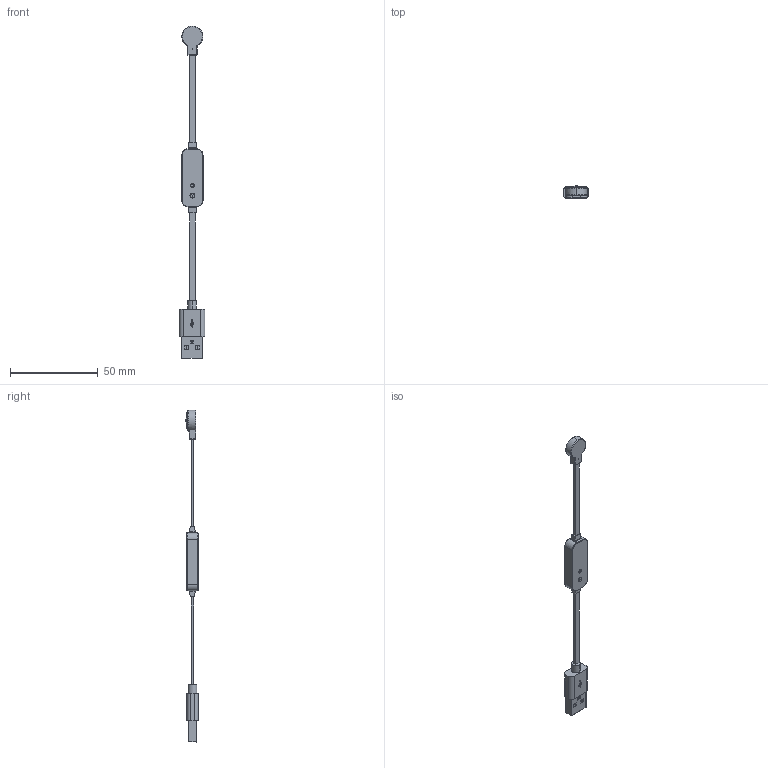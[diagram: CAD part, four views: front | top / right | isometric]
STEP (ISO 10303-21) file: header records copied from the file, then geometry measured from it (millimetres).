
FILE_DESCRIPTION (( 'STEP AP214' ), '1' );
FILE_NAME ('687N0222A011L2E.STEP', '2023-05-01T18:37:21', ( '' ), ( '' ), 'SwSTEP 2.0', 'SolidWorks 2020', '' );
FILE_SCHEMA (( 'AUTOMOTIVE_DESIGN' ));
Length unit declared in the file: millimetre
Products named in the file (1): 687N0222A011L2E
Bounding box: 14.6 x 7.29 x 189.51 mm (x, y, z)
Volume: 5597.2 mm3; surface area: 4721.9 mm2
Topology: 12 solids, 12 shells, 214 faces, 500 edges, 318 vertices
Faces by surface type: plane 132, cylinder 62, torus 14, sphere 6
Entity records: 6414 total; most frequent: DIRECTION 1061, CARTESIAN_POINT 1043, ORIENTED_EDGE 984, EDGE_CURVE 492, AXIS2_PLACEMENT_3D 358, LINE 345, VECTOR 345, VERTEX_POINT 316
